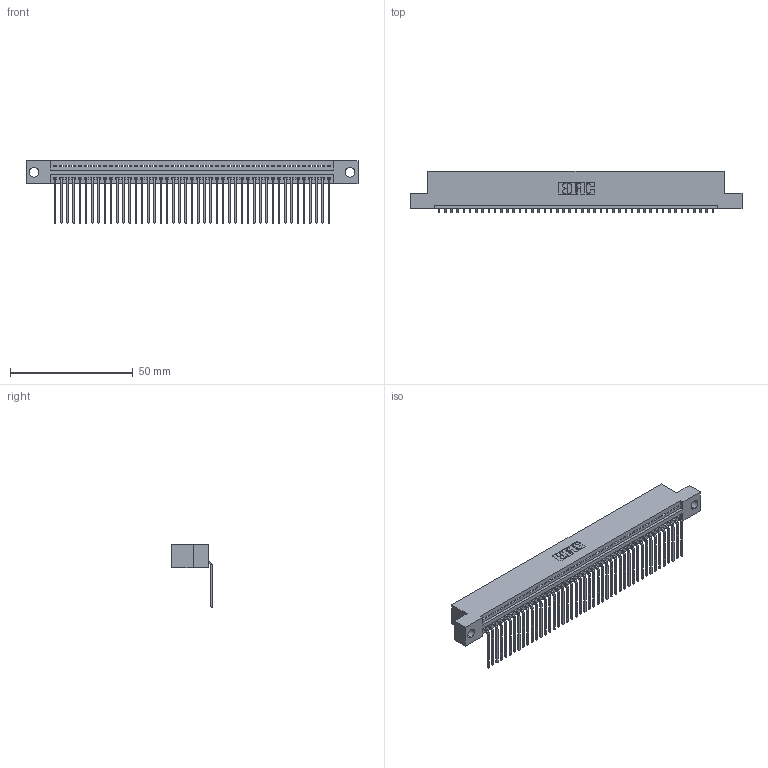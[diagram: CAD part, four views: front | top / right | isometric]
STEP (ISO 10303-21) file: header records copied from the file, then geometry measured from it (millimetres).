
FILE_DESCRIPTION (( 'STEP AP203' ), '1' );
FILE_NAME ('395-045-559-104.STEP', '2018-11-16T01:43:21', ( '' ), ( '' ), 'SwSTEP 2.0', 'SolidWorks 2016', '' );
FILE_SCHEMA (( 'CONFIG_CONTROL_DESIGN' ));
Length unit declared in the file: inch
Products named in the file (3): 345-292-001_558 559 Tail - 1; 395-045-559-104; 345 Part_Flush Mounting Lugs - 0.156 Dia-TH
Assembly tree (46 placements, depth 2):
  395-045-559-104
    345 Part_Flush Mounting Lugs - 0.156 Dia-TH
    345-292-001_558 559 Tail - 1  x45
Bounding box: 135.51 x 16.75 x 25.53 mm (x, y, z)
Volume: 12957.4 mm3; surface area: 17949.8 mm2
Topology: 46 solids, 46 shells, 2826 faces, 8531 edges, 5626 vertices
Faces by surface type: plane 1970, cylinder 856
Entity records: 33551 total; most frequent: CARTESIAN_POINT 5819, ORIENTED_EDGE 5798, DIRECTION 5077, EDGE_CURVE 2899, LINE 2587, VECTOR 2587, VERTEX_POINT 1930, AXIS2_PLACEMENT_3D 1245
